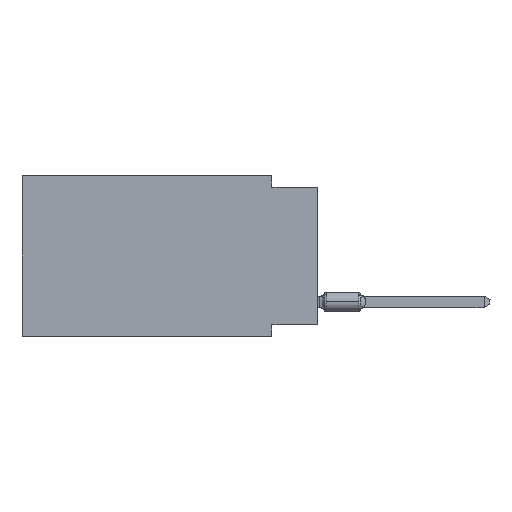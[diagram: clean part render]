
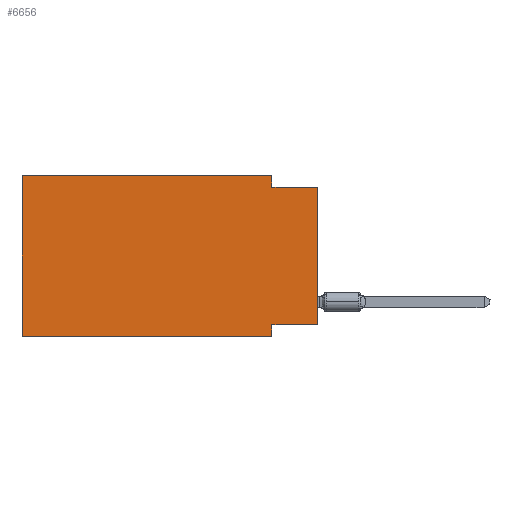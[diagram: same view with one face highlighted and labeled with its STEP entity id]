
A CAD part, left-side view. The second image highlights one B-rep face of the part: STEP entity #6656.
In plain terms, the highlighted planar face has unit normal (-1, 0, 0).
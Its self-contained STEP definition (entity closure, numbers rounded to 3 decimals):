
#251 = VERTEX_POINT ( 'NONE', #86591 ) ;
#2752 = DIRECTION ( 'NONE',  ( 0., 0., 1. ) ) ;
#4599 = VECTOR ( 'NONE', #45004, 1000. ) ;
#6656 = ADVANCED_FACE ( 'NONE', ( #51849 ), #102723, .F. ) ;
#6999 = EDGE_LOOP ( 'NONE', ( #99450, #40841, #64428, #28231, #15355, #25262, #66719, #109731 ) ) ;
#8689 = EDGE_CURVE ( 'NONE', #91414, #58207, #96560, .T. ) ;
#9063 = CARTESIAN_POINT ( 'NONE',  ( 0., 0., -8.255 ) ) ;
#10717 = CARTESIAN_POINT ( 'NONE',  ( 0., 2.54, -0.635 ) ) ;
#10729 = VECTOR ( 'NONE', #26989, 1000. ) ;
#14842 = DIRECTION ( 'NONE',  ( 0., 0., 1. ) ) ;
#15355 = ORIENTED_EDGE ( 'NONE', *, *, #25903, .F. ) ;
#18803 = VERTEX_POINT ( 'NONE', #9063 ) ;
#25081 = EDGE_CURVE ( 'NONE', #90531, #251, #78904, .T. ) ;
#25262 = ORIENTED_EDGE ( 'NONE', *, *, #76335, .T. ) ;
#25849 = DIRECTION ( 'NONE',  ( 1., 0., 0. ) ) ;
#25903 = EDGE_CURVE ( 'NONE', #37202, #91414, #98228, .T. ) ;
#26923 = EDGE_CURVE ( 'NONE', #18803, #251, #74193, .T. ) ;
#26989 = DIRECTION ( 'NONE',  ( 0., 0., -1. ) ) ;
#28148 = CARTESIAN_POINT ( 'NONE',  ( 0., 16.383, 0. ) ) ;
#28170 = CARTESIAN_POINT ( 'NONE',  ( 0., 16.383, 0. ) ) ;
#28231 = ORIENTED_EDGE ( 'NONE', *, *, #8689, .F. ) ;
#29340 = DIRECTION ( 'NONE',  ( 0., 0., -1. ) ) ;
#31134 = CARTESIAN_POINT ( 'NONE',  ( 0., 2.54, 0. ) ) ;
#37077 = DIRECTION ( 'NONE',  ( 0., -1., 0. ) ) ;
#37202 = VERTEX_POINT ( 'NONE', #41213 ) ;
#37848 = CARTESIAN_POINT ( 'NONE',  ( 0., 2.54, 0. ) ) ;
#38097 = VECTOR ( 'NONE', #111336, 1000. ) ;
#40841 = ORIENTED_EDGE ( 'NONE', *, *, #25081, .F. ) ;
#41213 = CARTESIAN_POINT ( 'NONE',  ( 0., 16.383, -8.89 ) ) ;
#43484 = EDGE_CURVE ( 'NONE', #106725, #90596, #69947, .T. ) ;
#44722 = VECTOR ( 'NONE', #14842, 1000. ) ;
#45004 = DIRECTION ( 'NONE',  ( 0., 1., 0. ) ) ;
#45560 = LINE ( 'NONE', #103809, #4599 ) ;
#47563 = CARTESIAN_POINT ( 'NONE',  ( 0., 16.383, 0. ) ) ;
#50054 = EDGE_CURVE ( 'NONE', #18803, #106725, #45560, .T. ) ;
#50216 = VECTOR ( 'NONE', #2752, 1000. ) ;
#51849 = FACE_OUTER_BOUND ( 'NONE', #6999, .T. ) ;
#52077 = VECTOR ( 'NONE', #97095, 1000. ) ;
#58207 = VERTEX_POINT ( 'NONE', #31134 ) ;
#61658 = EDGE_CURVE ( 'NONE', #58207, #90531, #63847, .T. ) ;
#63847 = LINE ( 'NONE', #37848, #76497 ) ;
#63860 = AXIS2_PLACEMENT_3D ( 'NONE', #103841, #25849, #86911 ) ;
#64428 = ORIENTED_EDGE ( 'NONE', *, *, #61658, .F. ) ;
#66719 = ORIENTED_EDGE ( 'NONE', *, *, #43484, .F. ) ;
#69947 = LINE ( 'NONE', #104422, #10729 ) ;
#74193 = LINE ( 'NONE', #92284, #44722 ) ;
#76335 = EDGE_CURVE ( 'NONE', #37202, #90596, #76873, .T. ) ;
#76497 = VECTOR ( 'NONE', #29340, 1000. ) ;
#76873 = LINE ( 'NONE', #90643, #38097 ) ;
#78904 = LINE ( 'NONE', #105995, #109674 ) ;
#86591 = CARTESIAN_POINT ( 'NONE',  ( 0., 0., -0.635 ) ) ;
#86911 = DIRECTION ( 'NONE',  ( 0., 0., -1. ) ) ;
#89257 = CARTESIAN_POINT ( 'NONE',  ( 0., 2.54, -8.89 ) ) ;
#90531 = VERTEX_POINT ( 'NONE', #10717 ) ;
#90596 = VERTEX_POINT ( 'NONE', #89257 ) ;
#90643 = CARTESIAN_POINT ( 'NONE',  ( 0., 16.383, -8.89 ) ) ;
#91414 = VERTEX_POINT ( 'NONE', #47563 ) ;
#92284 = CARTESIAN_POINT ( 'NONE',  ( 0., 0., 0. ) ) ;
#96560 = LINE ( 'NONE', #28148, #52077 ) ;
#97095 = DIRECTION ( 'NONE',  ( 0., -1., 0. ) ) ;
#98152 = CARTESIAN_POINT ( 'NONE',  ( 0., 2.54, -8.255 ) ) ;
#98228 = LINE ( 'NONE', #28170, #50216 ) ;
#99450 = ORIENTED_EDGE ( 'NONE', *, *, #26923, .T. ) ;
#102723 = PLANE ( 'NONE',  #63860 ) ;
#103809 = CARTESIAN_POINT ( 'NONE',  ( 0., 0., -8.255 ) ) ;
#103841 = CARTESIAN_POINT ( 'NONE',  ( 0., 16.383, 0. ) ) ;
#104422 = CARTESIAN_POINT ( 'NONE',  ( 0., 2.54, -8.89 ) ) ;
#105995 = CARTESIAN_POINT ( 'NONE',  ( 0., 0., -0.635 ) ) ;
#106725 = VERTEX_POINT ( 'NONE', #98152 ) ;
#109674 = VECTOR ( 'NONE', #37077, 1000. ) ;
#109731 = ORIENTED_EDGE ( 'NONE', *, *, #50054, .F. ) ;
#111336 = DIRECTION ( 'NONE',  ( 0., -1., 0. ) ) ;
